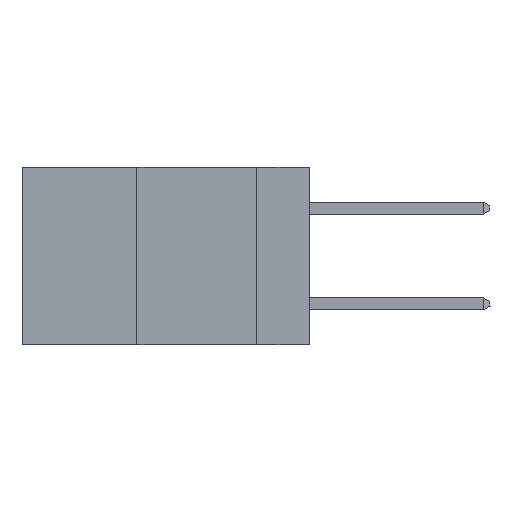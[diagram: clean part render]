
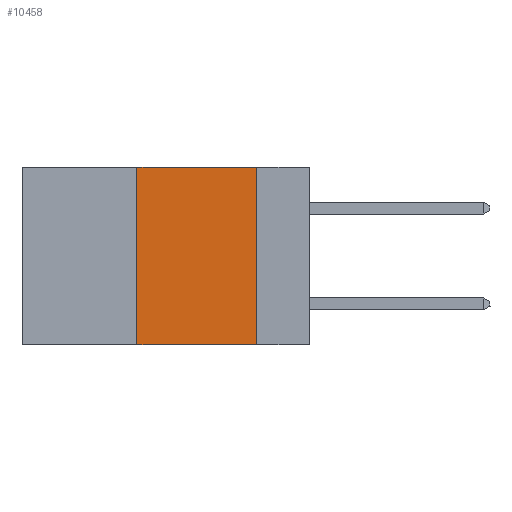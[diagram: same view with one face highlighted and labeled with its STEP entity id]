
A CAD part, left-side view. The second image highlights one B-rep face of the part: STEP entity #10458.
In plain terms, the highlighted planar face has unit normal (-1, 0, 0).
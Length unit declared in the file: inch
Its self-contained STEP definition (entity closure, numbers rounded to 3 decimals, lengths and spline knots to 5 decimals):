
#493 = ORIENTED_EDGE ( 'NONE', *, *, #16792, .F. ) ;
#869 = VERTEX_POINT ( 'NONE', #7061 ) ;
#1284 = DIRECTION ( 'NONE',  ( 0., -1., 0. ) ) ;
#1383 = CARTESIAN_POINT ( 'NONE',  ( 0., 0.6, 0. ) ) ;
#1826 = VECTOR ( 'NONE', #4063, 39.37008 ) ;
#1963 = CARTESIAN_POINT ( 'NONE',  ( 0., 0.11, 0. ) ) ;
#2037 = DIRECTION ( 'NONE',  ( 0., 0., -1. ) ) ;
#3490 = EDGE_CURVE ( 'NONE', #11660, #15514, #5499, .T. ) ;
#3681 = LINE ( 'NONE', #9050, #1826 ) ;
#3969 = CARTESIAN_POINT ( 'NONE',  ( 0., 0.6, -0.37 ) ) ;
#4063 = DIRECTION ( 'NONE',  ( 0., 0., 1. ) ) ;
#4121 = ORIENTED_EDGE ( 'NONE', *, *, #3490, .F. ) ;
#4342 = CARTESIAN_POINT ( 'NONE',  ( 0., 0.36, 0. ) ) ;
#5499 = LINE ( 'NONE', #6158, #11041 ) ;
#5808 = CARTESIAN_POINT ( 'NONE',  ( 0., 0.6, 0. ) ) ;
#6158 = CARTESIAN_POINT ( 'NONE',  ( 0., 0.11, 0. ) ) ;
#7061 = CARTESIAN_POINT ( 'NONE',  ( 0., 0.36, -0.37 ) ) ;
#7212 = VECTOR ( 'NONE', #10524, 39.37008 ) ;
#7286 = DIRECTION ( 'NONE',  ( 0., 0., -1. ) ) ;
#7935 = LINE ( 'NONE', #1383, #14244 ) ;
#8155 = EDGE_CURVE ( 'NONE', #869, #15514, #14957, .T. ) ;
#8783 = AXIS2_PLACEMENT_3D ( 'NONE', #5808, #14812, #2037 ) ;
#8828 = CARTESIAN_POINT ( 'NONE',  ( 0., 0.11, -0.37 ) ) ;
#9050 = CARTESIAN_POINT ( 'NONE',  ( 0., 0.36, 0. ) ) ;
#10458 = ADVANCED_FACE ( 'NONE', ( #13793 ), #12404, .F. ) ;
#10524 = DIRECTION ( 'NONE',  ( 0., -1., 0. ) ) ;
#11041 = VECTOR ( 'NONE', #7286, 39.37008 ) ;
#11281 = ORIENTED_EDGE ( 'NONE', *, *, #8155, .T. ) ;
#11660 = VERTEX_POINT ( 'NONE', #1963 ) ;
#12404 = PLANE ( 'NONE',  #8783 ) ;
#13418 = ORIENTED_EDGE ( 'NONE', *, *, #14377, .F. ) ;
#13793 = FACE_OUTER_BOUND ( 'NONE', #15012, .T. ) ;
#14244 = VECTOR ( 'NONE', #1284, 39.37008 ) ;
#14377 = EDGE_CURVE ( 'NONE', #14960, #11660, #7935, .T. ) ;
#14812 = DIRECTION ( 'NONE',  ( 1., 0., 0. ) ) ;
#14957 = LINE ( 'NONE', #3969, #7212 ) ;
#14960 = VERTEX_POINT ( 'NONE', #4342 ) ;
#15012 = EDGE_LOOP ( 'NONE', ( #4121, #13418, #493, #11281 ) ) ;
#15514 = VERTEX_POINT ( 'NONE', #8828 ) ;
#16792 = EDGE_CURVE ( 'NONE', #869, #14960, #3681, .T. ) ;
